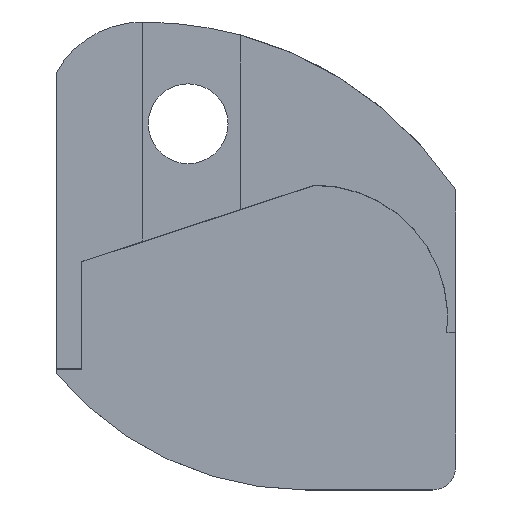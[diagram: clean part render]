
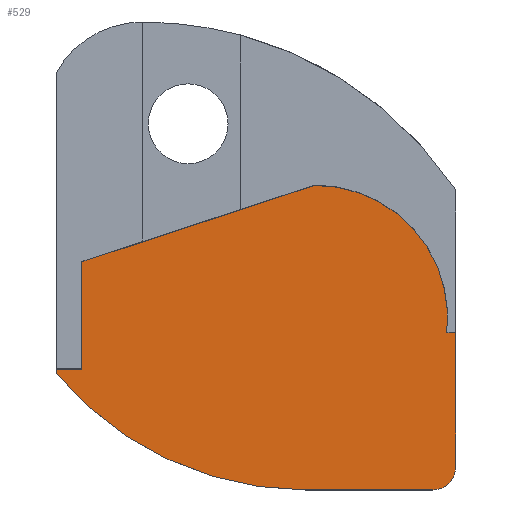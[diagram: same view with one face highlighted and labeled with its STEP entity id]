
A CAD part, top view. The second image highlights one B-rep face of the part: STEP entity #529.
In plain terms, the highlighted planar face has unit normal (0, 0, 1).
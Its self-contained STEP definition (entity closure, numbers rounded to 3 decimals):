
#28=PLANE('',#589);
#63=FACE_OUTER_BOUND('',#96,.T.);
#96=EDGE_LOOP('',(#426,#427,#428,#429,#430,#431,#432,#433,#434,#435));
#128=LINE('',#844,#180);
#133=LINE('',#856,#185);
#134=LINE('',#859,#186);
#135=LINE('',#863,#187);
#136=LINE('',#865,#188);
#137=LINE('',#867,#189);
#138=LINE('',#868,#190);
#180=VECTOR('',#683,10.);
#185=VECTOR('',#694,10.);
#186=VECTOR('',#697,10.);
#187=VECTOR('',#700,10.);
#188=VECTOR('',#701,10.);
#189=VECTOR('',#702,10.);
#190=VECTOR('',#703,10.);
#229=CIRCLE('',#584,14.227);
#230=CIRCLE('',#587,1.);
#231=CIRCLE('',#590,5.81);
#255=VERTEX_POINT('',#836);
#256=VERTEX_POINT('',#838);
#257=VERTEX_POINT('',#842);
#258=VERTEX_POINT('',#846);
#261=VERTEX_POINT('',#854);
#262=VERTEX_POINT('',#858);
#263=VERTEX_POINT('',#860);
#264=VERTEX_POINT('',#862);
#265=VERTEX_POINT('',#864);
#266=VERTEX_POINT('',#866);
#313=EDGE_CURVE('',#255,#256,#229,.T.);
#316=EDGE_CURVE('',#257,#255,#128,.T.);
#318=EDGE_CURVE('',#258,#257,#230,.T.);
#322=EDGE_CURVE('',#261,#258,#133,.T.);
#323=EDGE_CURVE('',#262,#261,#134,.T.);
#324=EDGE_CURVE('',#263,#262,#231,.T.);
#325=EDGE_CURVE('',#264,#263,#135,.T.);
#326=EDGE_CURVE('',#265,#264,#136,.T.);
#327=EDGE_CURVE('',#266,#265,#137,.T.);
#328=EDGE_CURVE('',#256,#266,#138,.T.);
#426=ORIENTED_EDGE('',*,*,#318,.F.);
#427=ORIENTED_EDGE('',*,*,#322,.F.);
#428=ORIENTED_EDGE('',*,*,#323,.F.);
#429=ORIENTED_EDGE('',*,*,#324,.F.);
#430=ORIENTED_EDGE('',*,*,#325,.F.);
#431=ORIENTED_EDGE('',*,*,#326,.F.);
#432=ORIENTED_EDGE('',*,*,#327,.F.);
#433=ORIENTED_EDGE('',*,*,#328,.F.);
#434=ORIENTED_EDGE('',*,*,#313,.F.);
#435=ORIENTED_EDGE('',*,*,#316,.F.);
#529=ADVANCED_FACE('',(#63),#28,.T.);
#584=AXIS2_PLACEMENT_3D('',#839,#677,#678);
#587=AXIS2_PLACEMENT_3D('',#848,#687,#688);
#589=AXIS2_PLACEMENT_3D('',#857,#695,#696);
#590=AXIS2_PLACEMENT_3D('',#861,#698,#699);
#677=DIRECTION('center_axis',(0.,0.,-1.));
#678=DIRECTION('ref_axis',(-0.768,-0.641,0.));
#683=DIRECTION('',(-1.,0.,0.));
#687=DIRECTION('center_axis',(0.,0.,-1.));
#688=DIRECTION('ref_axis',(0.707,-0.707,0.));
#694=DIRECTION('',(0.,-1.,0.));
#695=DIRECTION('center_axis',(0.,0.,1.));
#696=DIRECTION('ref_axis',(1.,0.,0.));
#697=DIRECTION('',(1.,0.,0.));
#698=DIRECTION('center_axis',(0.,0.,-1.));
#699=DIRECTION('ref_axis',(0.994,-0.11,0.));
#700=DIRECTION('',(0.95,0.313,0.));
#701=DIRECTION('',(0.,1.,0.));
#702=DIRECTION('',(1.,0.,0.));
#703=DIRECTION('',(0.,1.,0.));
#836=CARTESIAN_POINT('',(-6.579,1.9,-6.8));
#838=CARTESIAN_POINT('',(-17.5,7.01,-6.8));
#839=CARTESIAN_POINT('Origin',(-6.579,16.127,-6.8));
#842=CARTESIAN_POINT('',(-1.,1.9,-6.8));
#844=CARTESIAN_POINT('',(-4.375,1.9,-6.8));
#846=CARTESIAN_POINT('',(0.,2.9,-6.8));
#848=CARTESIAN_POINT('Origin',(-1.,2.9,-6.8));
#854=CARTESIAN_POINT('',(0.,8.8,-6.8));
#856=CARTESIAN_POINT('',(0.,11.338,-6.8));
#857=CARTESIAN_POINT('Origin',(-8.75,8.575,-6.8));
#858=CARTESIAN_POINT('',(-0.385,8.8,-6.8));
#859=CARTESIAN_POINT('',(-0.6,8.8,-6.8));
#860=CARTESIAN_POINT('',(-6.201,15.25,-6.8));
#861=CARTESIAN_POINT('Origin',(-6.16,9.44,-6.8));
#862=CARTESIAN_POINT('',(-16.378,11.897,-6.8));
#863=CARTESIAN_POINT('',(-16.378,11.897,-6.8));
#864=CARTESIAN_POINT('',(-16.378,7.2,-6.8));
#865=CARTESIAN_POINT('',(-16.378,11.397,-6.8));
#866=CARTESIAN_POINT('',(-17.5,7.2,-6.8));
#867=CARTESIAN_POINT('',(-16.378,7.2,-6.8));
#868=CARTESIAN_POINT('',(-17.5,7.792,-6.8));
